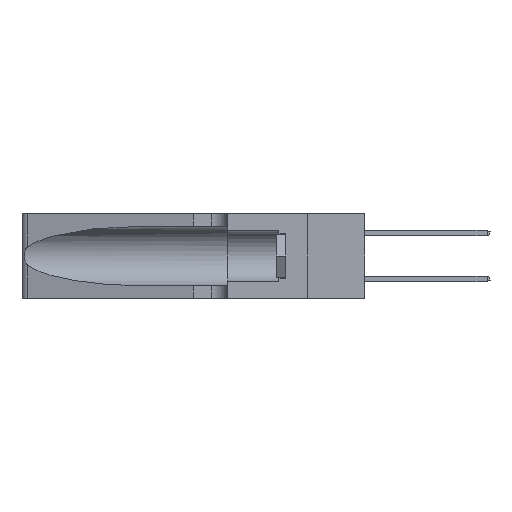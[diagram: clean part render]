
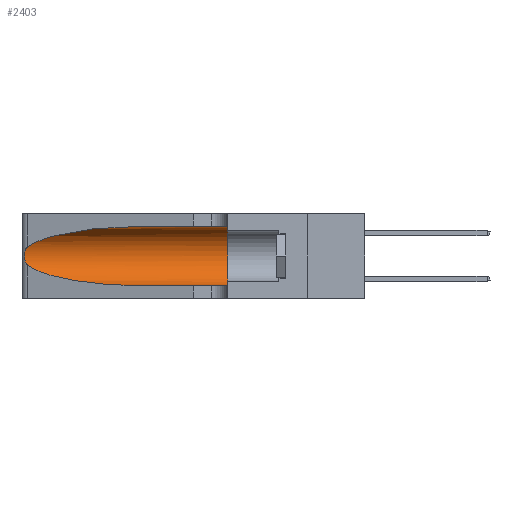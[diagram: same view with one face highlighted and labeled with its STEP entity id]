
A CAD part, left-side view. The second image highlights one B-rep face of the part: STEP entity #2403.
In plain terms, the highlighted cylindrical face has radius 3.308 mm (diameter 6.617 mm), a partial arc.
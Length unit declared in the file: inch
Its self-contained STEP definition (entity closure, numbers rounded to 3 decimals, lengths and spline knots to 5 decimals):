
#204 = B_SPLINE_CURVE_WITH_KNOTS ( 'NONE', 3,
 ( #7894, #18348, #644, #13265, #2479, #14996, #4295, #16735, #6116, #18422, #7975, #20118, #9778, #21822 ),
 .UNSPECIFIED., .F., .F.,
 ( 4, 2, 2, 2, 2, 2, 4 ),
 ( 0., 0.00027, 0.00053, 0.00107, 0.0016, 0.00187, 0.00214 ),
 .UNSPECIFIED. ) ;
#274 = LINE ( 'NONE', #2341, #5119 ) ;
#644 = CARTESIAN_POINT ( 'NONE',  ( 0.25639, 1.23184, 0.21858 ) ) ;
#909 = LINE ( 'NONE', #19832, #15765 ) ;
#974 = ORIENTED_EDGE ( 'NONE', *, *, #1124, .T. ) ;
#1124 = EDGE_CURVE ( 'NONE', #7050, #10728, #1244, .T. ) ;
#1215 = CARTESIAN_POINT ( 'NONE',  ( 0.18966, 0.96281, 0.05475 ) ) ;
#1244 =( BOUNDED_CURVE ( )  B_SPLINE_CURVE ( 3, ( #17712, #18293, #17041, #4305 ),
 .UNSPECIFIED., .F., .F. ) 
 B_SPLINE_CURVE_WITH_KNOTS ( ( 4, 4 ),
 ( 1.5708, 2.84003 ),
 .UNSPECIFIED. ) 
 CURVE ( )  GEOMETRIC_REPRESENTATION_ITEM ( )  RATIONAL_B_SPLINE_CURVE ( ( 1., 0.87, 0.87, 1. ) ) 
 REPRESENTATION_ITEM ( '' )  );
#2341 = CARTESIAN_POINT ( 'NONE',  ( 0.1305, 1.61858, 0.05475 ) ) ;
#2403 = ADVANCED_FACE ( 'NONE', ( #19953 ), #18888, .F. ) ;
#2479 = CARTESIAN_POINT ( 'NONE',  ( 0.25854, 1.2359, 0.20912 ) ) ;
#2645 = CARTESIAN_POINT ( 'NONE',  ( 0.25487, 1.22718, 0.22369 ) ) ;
#2976 = CARTESIAN_POINT ( 'NONE',  ( 0.1305, 0.72297, 0.05475 ) ) ;
#3162 = EDGE_CURVE ( 'NONE', #10728, #16398, #204, .T. ) ;
#4262 = ORIENTED_EDGE ( 'NONE', *, *, #16250, .F. ) ;
#4295 = CARTESIAN_POINT ( 'NONE',  ( 0.26075, 1.23896, 0.19203 ) ) ;
#4305 = CARTESIAN_POINT ( 'NONE',  ( 0.25487, 1.22718, 0.22369 ) ) ;
#4635 = VERTEX_POINT ( 'NONE', #13755 ) ;
#5119 = VECTOR ( 'NONE', #5908, 39.37008 ) ;
#5341 = ORIENTED_EDGE ( 'NONE', *, *, #9014, .T. ) ;
#5908 = DIRECTION ( 'NONE',  ( 0., -1., 0. ) ) ;
#6116 = CARTESIAN_POINT ( 'NONE',  ( 0.26017, 1.23833, 0.17102 ) ) ;
#6756 = EDGE_CURVE ( 'NONE', #13083, #4635, #17121, .T. ) ;
#7050 = VERTEX_POINT ( 'NONE', #15001 ) ;
#7369 = CARTESIAN_POINT ( 'NONE',  ( 0.1305, 0.35, 0.31525 ) ) ;
#7894 = CARTESIAN_POINT ( 'NONE',  ( 0.25487, 1.22718, 0.22369 ) ) ;
#7975 = CARTESIAN_POINT ( 'NONE',  ( 0.25789, 1.23486, 0.15765 ) ) ;
#8456 = CARTESIAN_POINT ( 'NONE',  ( 0.25487, 1.22718, 0.14631 ) ) ;
#9000 = CARTESIAN_POINT ( 'NONE',  ( 0.1305, 0.35, 0.185 ) ) ;
#9014 = EDGE_CURVE ( 'NONE', #17528, #4635, #274, .T. ) ;
#9064 = AXIS2_PLACEMENT_3D ( 'NONE', #9000, #21109, #10816 ) ;
#9227 = EDGE_CURVE ( 'NONE', #16398, #17528, #19514, .T. ) ;
#9725 = DIRECTION ( 'NONE',  ( 0., 0., -1. ) ) ;
#9778 = CARTESIAN_POINT ( 'NONE',  ( 0.25555, 1.22993, 0.14849 ) ) ;
#9832 = ORIENTED_EDGE ( 'NONE', *, *, #3162, .T. ) ;
#9948 = CARTESIAN_POINT ( 'NONE',  ( 0.25487, 1.22718, 0.14631 ) ) ;
#10062 = ORIENTED_EDGE ( 'NONE', *, *, #6756, .F. ) ;
#10728 = VERTEX_POINT ( 'NONE', #2645 ) ;
#10816 = DIRECTION ( 'NONE',  ( 0., 0., 1. ) ) ;
#11820 = EDGE_LOOP ( 'NONE', ( #974, #9832, #17454, #5341, #10062, #4262 ) ) ;
#13083 = VERTEX_POINT ( 'NONE', #7369 ) ;
#13265 = CARTESIAN_POINT ( 'NONE',  ( 0.25787, 1.23484, 0.2124 ) ) ;
#13755 = CARTESIAN_POINT ( 'NONE',  ( 0.1305, 0.35, 0.05475 ) ) ;
#13816 = CARTESIAN_POINT ( 'NONE',  ( 0.1305, 0.72297, 0.05475 ) ) ;
#14332 = AXIS2_PLACEMENT_3D ( 'NONE', #20074, #18379, #9725 ) ;
#14996 = CARTESIAN_POINT ( 'NONE',  ( 0.26018, 1.23835, 0.19895 ) ) ;
#15001 = CARTESIAN_POINT ( 'NONE',  ( 0.1305, 0.72297, 0.31525 ) ) ;
#15765 = VECTOR ( 'NONE', #16454, 39.37008 ) ;
#16250 = EDGE_CURVE ( 'NONE', #7050, #13083, #909, .T. ) ;
#16398 = VERTEX_POINT ( 'NONE', #9948 ) ;
#16454 = DIRECTION ( 'NONE',  ( 0., -1., 0. ) ) ;
#16735 = CARTESIAN_POINT ( 'NONE',  ( 0.26075, 1.23896, 0.178 ) ) ;
#17041 = CARTESIAN_POINT ( 'NONE',  ( 0.2373, 1.15595, 0.28018 ) ) ;
#17121 = CIRCLE ( 'NONE', #9064, 0.13025 ) ;
#17185 = CARTESIAN_POINT ( 'NONE',  ( 0.2373, 1.15595, 0.08982 ) ) ;
#17454 = ORIENTED_EDGE ( 'NONE', *, *, #9227, .T. ) ;
#17528 = VERTEX_POINT ( 'NONE', #2976 ) ;
#17712 = CARTESIAN_POINT ( 'NONE',  ( 0.1305, 0.72297, 0.31525 ) ) ;
#18293 = CARTESIAN_POINT ( 'NONE',  ( 0.18966, 0.96281, 0.31525 ) ) ;
#18348 = CARTESIAN_POINT ( 'NONE',  ( 0.25555, 1.22994, 0.2215 ) ) ;
#18379 = DIRECTION ( 'NONE',  ( 0., -1., 0. ) ) ;
#18422 = CARTESIAN_POINT ( 'NONE',  ( 0.25856, 1.23593, 0.16098 ) ) ;
#18888 = CYLINDRICAL_SURFACE ( 'NONE', #14332, 0.13025 ) ;
#19514 =( BOUNDED_CURVE ( )  B_SPLINE_CURVE ( 3, ( #8456, #17185, #1215, #13816 ),
 .UNSPECIFIED., .F., .T. ) 
 B_SPLINE_CURVE_WITH_KNOTS ( ( 4, 4 ),
 ( 3.44316, 4.71239 ),
 .UNSPECIFIED. ) 
 CURVE ( )  GEOMETRIC_REPRESENTATION_ITEM ( )  RATIONAL_B_SPLINE_CURVE ( ( 1., 0.87, 0.87, 1. ) ) 
 REPRESENTATION_ITEM ( '' )  );
#19832 = CARTESIAN_POINT ( 'NONE',  ( 0.1305, 1.61858, 0.31525 ) ) ;
#19953 = FACE_OUTER_BOUND ( 'NONE', #11820, .T. ) ;
#20074 = CARTESIAN_POINT ( 'NONE',  ( 0.1305, 1.61858, 0.185 ) ) ;
#20118 = CARTESIAN_POINT ( 'NONE',  ( 0.25639, 1.23186, 0.15144 ) ) ;
#21109 = DIRECTION ( 'NONE',  ( 0., 1., 0. ) ) ;
#21822 = CARTESIAN_POINT ( 'NONE',  ( 0.25487, 1.22718, 0.14631 ) ) ;
